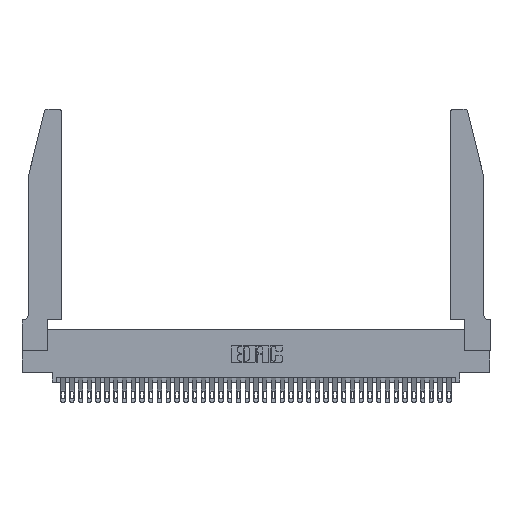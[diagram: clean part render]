
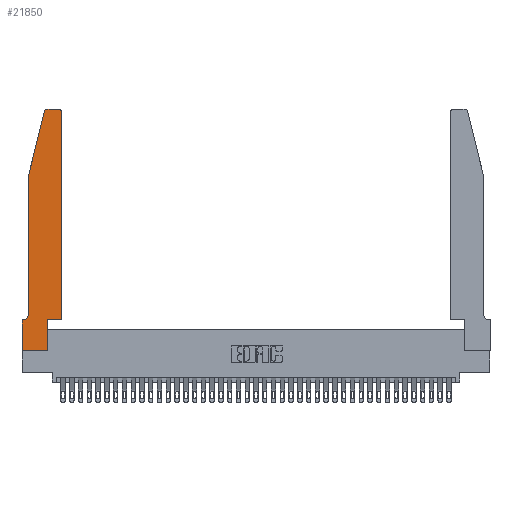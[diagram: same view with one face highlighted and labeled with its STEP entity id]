
A CAD part, top view. The second image highlights one B-rep face of the part: STEP entity #21850.
In plain terms, the highlighted planar face has unit normal (0, 0, 1).
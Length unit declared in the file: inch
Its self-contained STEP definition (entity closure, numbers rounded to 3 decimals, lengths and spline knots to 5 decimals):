
#608 = VECTOR ( 'NONE', #24120, 39.37008 ) ;
#1161 = ORIENTED_EDGE ( 'NONE', *, *, #16800, .T. ) ;
#1803 = PLANE ( 'NONE',  #26028 ) ;
#2046 = ORIENTED_EDGE ( 'NONE', *, *, #30790, .T. ) ;
#2174 = EDGE_CURVE ( 'NONE', #39708, #28948, #36498, .T. ) ;
#2378 = VECTOR ( 'NONE', #35331, 39.37008 ) ;
#2721 = CARTESIAN_POINT ( 'NONE',  ( 0.0755, 2., 0.37 ) ) ;
#2922 = DIRECTION ( 'NONE',  ( 1., 0., 0. ) ) ;
#3057 = LINE ( 'NONE', #8526, #608 ) ;
#3746 = DIRECTION ( 'NONE',  ( 1., 0., 0. ) ) ;
#4910 = DIRECTION ( 'NONE',  ( 1., 0., 0. ) ) ;
#5294 = CARTESIAN_POINT ( 'NONE',  ( 0.0755, 2., 0.37 ) ) ;
#5491 = VERTEX_POINT ( 'NONE', #23738 ) ;
#5672 = EDGE_CURVE ( 'NONE', #34185, #7940, #40138, .T. ) ;
#5856 = VERTEX_POINT ( 'NONE', #21544 ) ;
#7411 = VECTOR ( 'NONE', #25731, 39.37008 ) ;
#7940 = VERTEX_POINT ( 'NONE', #31627 ) ;
#8085 = ORIENTED_EDGE ( 'NONE', *, *, #37085, .T. ) ;
#8526 = CARTESIAN_POINT ( 'NONE',  ( 0., 0., 0.37 ) ) ;
#8821 = ORIENTED_EDGE ( 'NONE', *, *, #27306, .T. ) ;
#9019 = EDGE_CURVE ( 'NONE', #20875, #34185, #38765, .T. ) ;
#9549 = VECTOR ( 'NONE', #3746, 39.37008 ) ;
#9635 = AXIS2_PLACEMENT_3D ( 'NONE', #34028, #36915, #2922 ) ;
#10134 = CARTESIAN_POINT ( 'NONE',  ( 0.4505, 2.72, 0.37 ) ) ;
#10743 = DIRECTION ( 'NONE',  ( 0., 0., 1. ) ) ;
#10884 = CARTESIAN_POINT ( 'NONE',  ( 0.2605, 2.75, 0.37 ) ) ;
#10923 = ORIENTED_EDGE ( 'NONE', *, *, #23284, .T. ) ;
#11470 = DIRECTION ( 'NONE',  ( 0., 0., 1. ) ) ;
#11587 = ORIENTED_EDGE ( 'NONE', *, *, #30993, .T. ) ;
#13275 = CARTESIAN_POINT ( 'NONE',  ( 0., 0., 0.37 ) ) ;
#13473 = LINE ( 'NONE', #13275, #9549 ) ;
#14132 = ORIENTED_EDGE ( 'NONE', *, *, #2174, .T. ) ;
#14171 = CIRCLE ( 'NONE', #9635, 0.03 ) ;
#14741 = DIRECTION ( 'NONE',  ( 1., 0., 0. ) ) ;
#14829 = DIRECTION ( 'NONE',  ( 0., -1., 0. ) ) ;
#14958 = CIRCLE ( 'NONE', #32352, 0.03 ) ;
#16309 = CARTESIAN_POINT ( 'NONE',  ( 0.0755, 0.42, 0.37 ) ) ;
#16800 = EDGE_CURVE ( 'NONE', #24704, #39708, #18552, .T. ) ;
#17472 = DIRECTION ( 'NONE',  ( -1., 0., 0. ) ) ;
#17912 = CARTESIAN_POINT ( 'NONE',  ( 0., 0.35, 0.37 ) ) ;
#18410 = CARTESIAN_POINT ( 'NONE',  ( 0.2865, 0., 0.37 ) ) ;
#18552 = LINE ( 'NONE', #5294, #36450 ) ;
#19026 = VECTOR ( 'NONE', #33072, 39.37008 ) ;
#19250 = CARTESIAN_POINT ( 'NONE',  ( 0.0755, 0.35, 0.37 ) ) ;
#20060 = LINE ( 'NONE', #19250, #7411 ) ;
#20173 = DIRECTION ( 'NONE',  ( 0., 0., -1. ) ) ;
#20203 = CARTESIAN_POINT ( 'NONE',  ( 0.4505, 0.35, 0.37 ) ) ;
#20875 = VERTEX_POINT ( 'NONE', #18410 ) ;
#20910 = CARTESIAN_POINT ( 'NONE',  ( 0.284, 2.75, 0.37 ) ) ;
#21544 = CARTESIAN_POINT ( 'NONE',  ( 0.4205, 2.75, 0.37 ) ) ;
#21776 = LINE ( 'NONE', #38415, #31863 ) ;
#21850 = ADVANCED_FACE ( 'NONE', ( #39866 ), #1803, .T. ) ;
#21944 = VERTEX_POINT ( 'NONE', #20910 ) ;
#21978 = CARTESIAN_POINT ( 'NONE',  ( 0.2865, 0.35, 0.37 ) ) ;
#22044 = CARTESIAN_POINT ( 'NONE',  ( 0.0755, 2., 0.37 ) ) ;
#22391 = ORIENTED_EDGE ( 'NONE', *, *, #31770, .T. ) ;
#22740 = LINE ( 'NONE', #22044, #2378 ) ;
#23252 = DIRECTION ( 'NONE',  ( 0., 1., 0. ) ) ;
#23284 = EDGE_CURVE ( 'NONE', #30421, #24704, #22740, .T. ) ;
#23331 = ORIENTED_EDGE ( 'NONE', *, *, #27324, .T. ) ;
#23598 = DIRECTION ( 'NONE',  ( 1., 0., 0. ) ) ;
#23700 = ORIENTED_EDGE ( 'NONE', *, *, #25012, .T. ) ;
#23738 = CARTESIAN_POINT ( 'NONE',  ( 0., 0., 0.37 ) ) ;
#23910 = LINE ( 'NONE', #10884, #19026 ) ;
#24120 = DIRECTION ( 'NONE',  ( 0., -1., 0. ) ) ;
#24704 = VERTEX_POINT ( 'NONE', #2721 ) ;
#25012 = EDGE_CURVE ( 'NONE', #5491, #20875, #13473, .T. ) ;
#25731 = DIRECTION ( 'NONE',  ( -1., 0., 0. ) ) ;
#26028 = AXIS2_PLACEMENT_3D ( 'NONE', #29707, #10743, #4910 ) ;
#26133 = VECTOR ( 'NONE', #34712, 39.37008 ) ;
#27306 = EDGE_CURVE ( 'NONE', #7940, #34407, #21776, .T. ) ;
#27324 = EDGE_CURVE ( 'NONE', #21944, #30421, #14958, .T. ) ;
#27534 = VECTOR ( 'NONE', #23598, 39.37008 ) ;
#28108 = VERTEX_POINT ( 'NONE', #17912 ) ;
#28661 = CARTESIAN_POINT ( 'NONE',  ( 0.0055, 0.35, 0.37 ) ) ;
#28948 = VERTEX_POINT ( 'NONE', #28661 ) ;
#29707 = CARTESIAN_POINT ( 'NONE',  ( 0., 0.35, 0.37 ) ) ;
#30421 = VERTEX_POINT ( 'NONE', #40001 ) ;
#30790 = EDGE_CURVE ( 'NONE', #28948, #28108, #20060, .T. ) ;
#30993 = EDGE_CURVE ( 'NONE', #28108, #5491, #3057, .T. ) ;
#31000 = CARTESIAN_POINT ( 'NONE',  ( 0.2865, 0.35, 0.37 ) ) ;
#31627 = CARTESIAN_POINT ( 'NONE',  ( 0.4505, 0.35, 0.37 ) ) ;
#31770 = EDGE_CURVE ( 'NONE', #34407, #5856, #14171, .T. ) ;
#31863 = VECTOR ( 'NONE', #23252, 39.37008 ) ;
#31908 = CARTESIAN_POINT ( 'NONE',  ( 0.0055, 0.42, 0.37 ) ) ;
#32352 = AXIS2_PLACEMENT_3D ( 'NONE', #33363, #11470, #14741 ) ;
#32866 = AXIS2_PLACEMENT_3D ( 'NONE', #31908, #20173, #17472 ) ;
#33072 = DIRECTION ( 'NONE',  ( -1., 0., 0. ) ) ;
#33148 = ORIENTED_EDGE ( 'NONE', *, *, #5672, .T. ) ;
#33363 = CARTESIAN_POINT ( 'NONE',  ( 0.284, 2.72, 0.37 ) ) ;
#34028 = CARTESIAN_POINT ( 'NONE',  ( 0.4205, 2.72, 0.37 ) ) ;
#34185 = VERTEX_POINT ( 'NONE', #31000 ) ;
#34407 = VERTEX_POINT ( 'NONE', #10134 ) ;
#34712 = DIRECTION ( 'NONE',  ( 0., 1., 0. ) ) ;
#35331 = DIRECTION ( 'NONE',  ( -0.239, -0.971, 0. ) ) ;
#36450 = VECTOR ( 'NONE', #14829, 39.37008 ) ;
#36498 = CIRCLE ( 'NONE', #32866, 0.07 ) ;
#36915 = DIRECTION ( 'NONE',  ( 0., 0., 1. ) ) ;
#37085 = EDGE_CURVE ( 'NONE', #5856, #21944, #23910, .T. ) ;
#37673 = EDGE_LOOP ( 'NONE', ( #8085, #23331, #10923, #1161, #14132, #2046, #11587, #23700, #39609, #33148, #8821, #22391 ) ) ;
#38415 = CARTESIAN_POINT ( 'NONE',  ( 0.4505, 0.35, 0.37 ) ) ;
#38765 = LINE ( 'NONE', #21978, #26133 ) ;
#39609 = ORIENTED_EDGE ( 'NONE', *, *, #9019, .T. ) ;
#39708 = VERTEX_POINT ( 'NONE', #16309 ) ;
#39866 = FACE_OUTER_BOUND ( 'NONE', #37673, .T. ) ;
#40001 = CARTESIAN_POINT ( 'NONE',  ( 0.25487, 2.72718, 0.37 ) ) ;
#40138 = LINE ( 'NONE', #20203, #27534 ) ;
